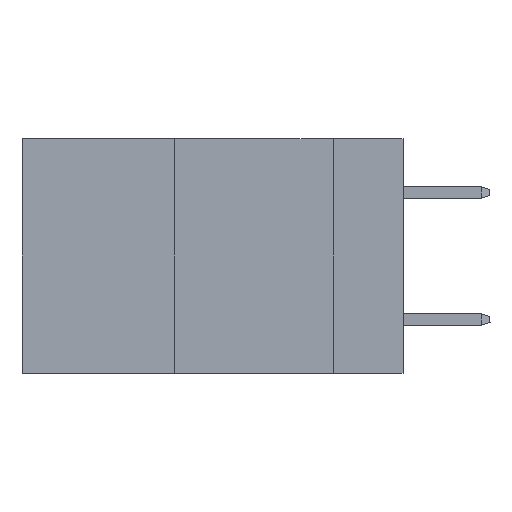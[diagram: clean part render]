
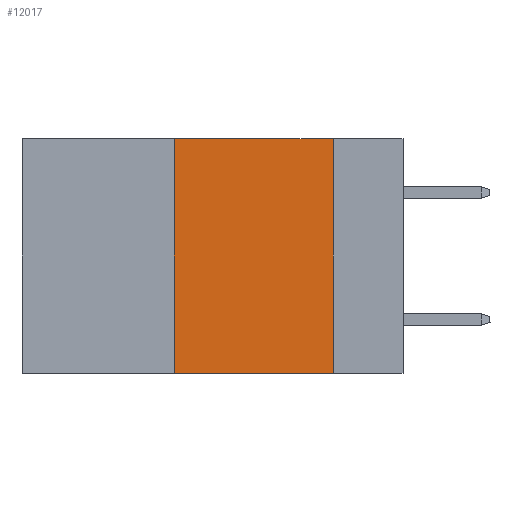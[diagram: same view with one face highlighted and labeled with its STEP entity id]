
A CAD part, left-side view. The second image highlights one B-rep face of the part: STEP entity #12017.
In plain terms, the highlighted planar face has unit normal (-1, 0, 0).
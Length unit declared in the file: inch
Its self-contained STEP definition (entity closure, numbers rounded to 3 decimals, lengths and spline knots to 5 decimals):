
#486 = LINE ( 'NONE', #4284, #13237 ) ;
#797 = CARTESIAN_POINT ( 'NONE',  ( 0., 0.11, 0. ) ) ;
#2446 = DIRECTION ( 'NONE',  ( 0., 0., -1. ) ) ;
#3340 = LINE ( 'NONE', #3696, #6061 ) ;
#3696 = CARTESIAN_POINT ( 'NONE',  ( 0., 0.6, -0.37 ) ) ;
#4282 = FACE_OUTER_BOUND ( 'NONE', #17143, .T. ) ;
#4284 = CARTESIAN_POINT ( 'NONE',  ( 0., 0.6, 0. ) ) ;
#4559 = EDGE_CURVE ( 'NONE', #9863, #14832, #19579, .T. ) ;
#4600 = DIRECTION ( 'NONE',  ( 0., 0., -1. ) ) ;
#5408 = ORIENTED_EDGE ( 'NONE', *, *, #6977, .T. ) ;
#5888 = ORIENTED_EDGE ( 'NONE', *, *, #13307, .F. ) ;
#6061 = VECTOR ( 'NONE', #15237, 39.37008 ) ;
#6580 = CARTESIAN_POINT ( 'NONE',  ( 0., 0.11, -0.37 ) ) ;
#6977 = EDGE_CURVE ( 'NONE', #20169, #14832, #3340, .T. ) ;
#9863 = VERTEX_POINT ( 'NONE', #15911 ) ;
#11390 = EDGE_CURVE ( 'NONE', #20169, #19717, #21393, .T. ) ;
#11441 = CARTESIAN_POINT ( 'NONE',  ( 0., 0.36, 0. ) ) ;
#11576 = PLANE ( 'NONE',  #14839 ) ;
#12017 = ADVANCED_FACE ( 'NONE', ( #4282 ), #11576, .F. ) ;
#12862 = VECTOR ( 'NONE', #18336, 39.37008 ) ;
#13237 = VECTOR ( 'NONE', #15483, 39.37008 ) ;
#13307 = EDGE_CURVE ( 'NONE', #19717, #9863, #486, .T. ) ;
#13976 = DIRECTION ( 'NONE',  ( 1., 0., 0. ) ) ;
#14832 = VERTEX_POINT ( 'NONE', #6580 ) ;
#14839 = AXIS2_PLACEMENT_3D ( 'NONE', #19016, #13976, #2446 ) ;
#15237 = DIRECTION ( 'NONE',  ( 0., -1., 0. ) ) ;
#15483 = DIRECTION ( 'NONE',  ( 0., -1., 0. ) ) ;
#15659 = VECTOR ( 'NONE', #4600, 39.37008 ) ;
#15911 = CARTESIAN_POINT ( 'NONE',  ( 0., 0.11, 0. ) ) ;
#16638 = CARTESIAN_POINT ( 'NONE',  ( 0., 0.36, 0. ) ) ;
#17143 = EDGE_LOOP ( 'NONE', ( #21504, #5888, #19866, #5408 ) ) ;
#18336 = DIRECTION ( 'NONE',  ( 0., 0., 1. ) ) ;
#19016 = CARTESIAN_POINT ( 'NONE',  ( 0., 0.6, 0. ) ) ;
#19579 = LINE ( 'NONE', #797, #15659 ) ;
#19717 = VERTEX_POINT ( 'NONE', #11441 ) ;
#19792 = CARTESIAN_POINT ( 'NONE',  ( 0., 0.36, -0.37 ) ) ;
#19866 = ORIENTED_EDGE ( 'NONE', *, *, #11390, .F. ) ;
#20169 = VERTEX_POINT ( 'NONE', #19792 ) ;
#21393 = LINE ( 'NONE', #16638, #12862 ) ;
#21504 = ORIENTED_EDGE ( 'NONE', *, *, #4559, .F. ) ;
